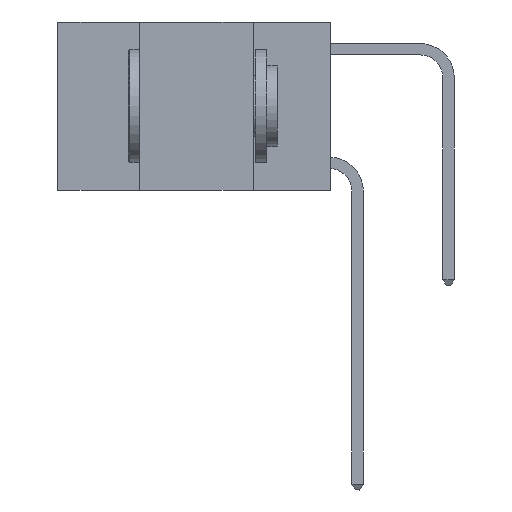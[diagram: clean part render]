
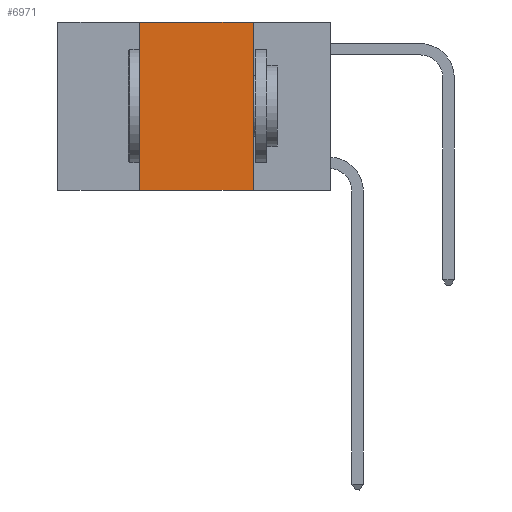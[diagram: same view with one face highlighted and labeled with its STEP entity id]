
A CAD part, left-side view. The second image highlights one B-rep face of the part: STEP entity #6971.
In plain terms, the highlighted planar face has unit normal (-1, 0, 0).
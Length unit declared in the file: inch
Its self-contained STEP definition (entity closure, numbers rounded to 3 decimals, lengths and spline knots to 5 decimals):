
#801 = DIRECTION ( 'NONE',  ( 0., -1., 0. ) ) ;
#1836 = CARTESIAN_POINT ( 'NONE',  ( 0., 0.17, -0.37 ) ) ;
#2915 = VECTOR ( 'NONE', #13041, 39.37008 ) ;
#3001 = PLANE ( 'NONE',  #16063 ) ;
#3471 = CARTESIAN_POINT ( 'NONE',  ( 0., 0.42, 0. ) ) ;
#3527 = LINE ( 'NONE', #4583, #15226 ) ;
#3544 = CARTESIAN_POINT ( 'NONE',  ( 0., 0.42, -0.37 ) ) ;
#3588 = LINE ( 'NONE', #16136, #20526 ) ;
#4583 = CARTESIAN_POINT ( 'NONE',  ( 0., 0.6, -0.37 ) ) ;
#6179 = CARTESIAN_POINT ( 'NONE',  ( 0., 0.6, 0. ) ) ;
#6506 = DIRECTION ( 'NONE',  ( 0., 0., -1. ) ) ;
#6574 = VECTOR ( 'NONE', #801, 39.37008 ) ;
#6971 = ADVANCED_FACE ( 'NONE', ( #12915 ), #3001, .F. ) ;
#7424 = ORIENTED_EDGE ( 'NONE', *, *, #12791, .F. ) ;
#7556 = CARTESIAN_POINT ( 'NONE',  ( 0., 0.17, 0. ) ) ;
#7728 = DIRECTION ( 'NONE',  ( 1., 0., 0. ) ) ;
#8016 = EDGE_CURVE ( 'NONE', #20240, #8230, #10762, .T. ) ;
#8230 = VERTEX_POINT ( 'NONE', #7556 ) ;
#8477 = VERTEX_POINT ( 'NONE', #1836 ) ;
#9194 = EDGE_CURVE ( 'NONE', #8230, #8477, #3588, .T. ) ;
#9242 = VERTEX_POINT ( 'NONE', #3544 ) ;
#10418 = ORIENTED_EDGE ( 'NONE', *, *, #16526, .T. ) ;
#10762 = LINE ( 'NONE', #16655, #6574 ) ;
#11238 = ORIENTED_EDGE ( 'NONE', *, *, #9194, .F. ) ;
#11291 = LINE ( 'NONE', #3471, #2915 ) ;
#12791 = EDGE_CURVE ( 'NONE', #9242, #20240, #11291, .T. ) ;
#12915 = FACE_OUTER_BOUND ( 'NONE', #19683, .T. ) ;
#13041 = DIRECTION ( 'NONE',  ( 0., 0., 1. ) ) ;
#13342 = ORIENTED_EDGE ( 'NONE', *, *, #8016, .F. ) ;
#15226 = VECTOR ( 'NONE', #15975, 39.37008 ) ;
#15975 = DIRECTION ( 'NONE',  ( 0., -1., 0. ) ) ;
#16063 = AXIS2_PLACEMENT_3D ( 'NONE', #6179, #7728, #18924 ) ;
#16136 = CARTESIAN_POINT ( 'NONE',  ( 0., 0.17, 0. ) ) ;
#16526 = EDGE_CURVE ( 'NONE', #9242, #8477, #3527, .T. ) ;
#16655 = CARTESIAN_POINT ( 'NONE',  ( 0., 0.6, 0. ) ) ;
#17344 = CARTESIAN_POINT ( 'NONE',  ( 0., 0.42, 0. ) ) ;
#18924 = DIRECTION ( 'NONE',  ( 0., 0., -1. ) ) ;
#19683 = EDGE_LOOP ( 'NONE', ( #11238, #13342, #7424, #10418 ) ) ;
#20240 = VERTEX_POINT ( 'NONE', #17344 ) ;
#20526 = VECTOR ( 'NONE', #6506, 39.37008 ) ;
